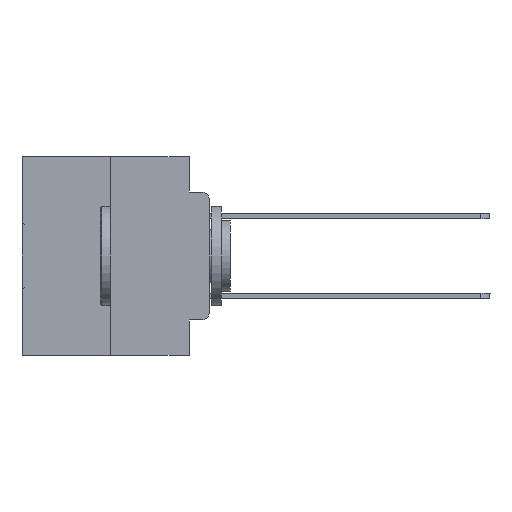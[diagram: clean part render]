
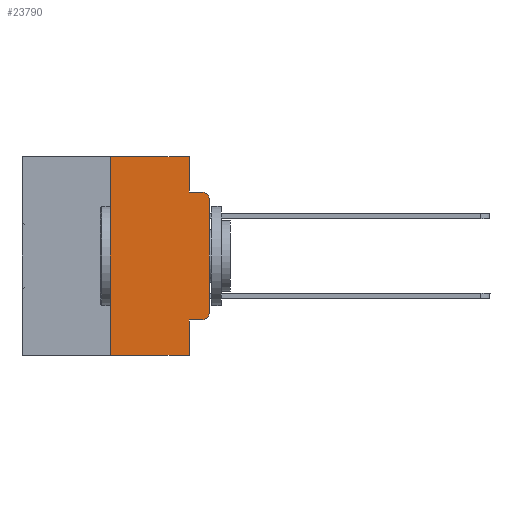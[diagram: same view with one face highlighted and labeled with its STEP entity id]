
A CAD part, left-side view. The second image highlights one B-rep face of the part: STEP entity #23790.
In plain terms, the highlighted planar face has unit normal (-1, 0, 0).
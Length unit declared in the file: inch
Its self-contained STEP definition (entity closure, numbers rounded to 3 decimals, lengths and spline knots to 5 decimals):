
#3 = VERTEX_POINT ( 'NONE', #14954 ) ;
#69 = ORIENTED_EDGE ( 'NONE', *, *, #8467, .T. ) ;
#255 = CARTESIAN_POINT ( 'NONE',  ( 0., 0.25, 0. ) ) ;
#316 = CARTESIAN_POINT ( 'NONE',  ( 0., 0.02, -0.3915 ) ) ;
#676 = EDGE_CURVE ( 'NONE', #5195, #7678, #20187, .T. ) ;
#709 = CARTESIAN_POINT ( 'NONE',  ( 0., 0.02, -0.0885 ) ) ;
#1615 = LINE ( 'NONE', #7010, #13814 ) ;
#2906 = VECTOR ( 'NONE', #10260, 39.37008 ) ;
#2927 = CARTESIAN_POINT ( 'NONE',  ( 0., 0.051, -0.4115 ) ) ;
#3789 = AXIS2_PLACEMENT_3D ( 'NONE', #316, #27270, #6475 ) ;
#3833 = DIRECTION ( 'NONE',  ( 1., 0., 0. ) ) ;
#3973 = EDGE_CURVE ( 'NONE', #9567, #18246, #27916, .T. ) ;
#4090 = EDGE_CURVE ( 'NONE', #33981, #18246, #19325, .T. ) ;
#4239 = EDGE_LOOP ( 'NONE', ( #30307, #14714, #23912, #22404, #26492, #5807, #30471, #18160, #69, #4255 ) ) ;
#4255 = ORIENTED_EDGE ( 'NONE', *, *, #676, .T. ) ;
#5195 = VERTEX_POINT ( 'NONE', #33158 ) ;
#5348 = LINE ( 'NONE', #20904, #2906 ) ;
#5396 = AXIS2_PLACEMENT_3D ( 'NONE', #18741, #26130, #15619 ) ;
#5807 = ORIENTED_EDGE ( 'NONE', *, *, #30444, .F. ) ;
#5916 = CARTESIAN_POINT ( 'NONE',  ( 0., 0.473, 0. ) ) ;
#6094 = DIRECTION ( 'NONE',  ( 0., 0., -1. ) ) ;
#6273 = EDGE_CURVE ( 'NONE', #7678, #33981, #1615, .T. ) ;
#6424 = CARTESIAN_POINT ( 'NONE',  ( 0., 0., -0.1085 ) ) ;
#6475 = DIRECTION ( 'NONE',  ( 0., 0., -1. ) ) ;
#7010 = CARTESIAN_POINT ( 'NONE',  ( 0., 0., 0. ) ) ;
#7244 = CARTESIAN_POINT ( 'NONE',  ( 0., 0.051, 0. ) ) ;
#7501 = LINE ( 'NONE', #28876, #15876 ) ;
#7605 = DIRECTION ( 'NONE',  ( 0., 0., 1. ) ) ;
#7678 = VERTEX_POINT ( 'NONE', #19292 ) ;
#8467 = EDGE_CURVE ( 'NONE', #31518, #5195, #26892, .T. ) ;
#8508 = CARTESIAN_POINT ( 'NONE',  ( 0., 0.051, -0.4115 ) ) ;
#9567 = VERTEX_POINT ( 'NONE', #23445 ) ;
#10260 = DIRECTION ( 'NONE',  ( 0., -1., 0. ) ) ;
#10972 = DIRECTION ( 'NONE',  ( 0., -1., 0. ) ) ;
#11409 = VECTOR ( 'NONE', #33988, 39.37008 ) ;
#11615 = VERTEX_POINT ( 'NONE', #28752 ) ;
#12507 = VECTOR ( 'NONE', #20404, 39.37008 ) ;
#12543 = CARTESIAN_POINT ( 'NONE',  ( 0., 0.051, 0. ) ) ;
#12655 = AXIS2_PLACEMENT_3D ( 'NONE', #5916, #3833, #6094 ) ;
#12841 = CARTESIAN_POINT ( 'NONE',  ( 0., 0.051, -0.5 ) ) ;
#13814 = VECTOR ( 'NONE', #17333, 39.37008 ) ;
#14016 = EDGE_CURVE ( 'NONE', #11615, #25646, #5348, .T. ) ;
#14714 = ORIENTED_EDGE ( 'NONE', *, *, #4090, .T. ) ;
#14954 = CARTESIAN_POINT ( 'NONE',  ( 0., 0.25, -0.5 ) ) ;
#15427 = VECTOR ( 'NONE', #20348, 39.37008 ) ;
#15507 = VECTOR ( 'NONE', #10972, 39.37008 ) ;
#15619 = DIRECTION ( 'NONE',  ( 0., 0., -1. ) ) ;
#15876 = VECTOR ( 'NONE', #29047, 39.37008 ) ;
#17333 = DIRECTION ( 'NONE',  ( 0., 0., 1. ) ) ;
#18160 = ORIENTED_EDGE ( 'NONE', *, *, #18769, .F. ) ;
#18246 = VERTEX_POINT ( 'NONE', #709 ) ;
#18741 = CARTESIAN_POINT ( 'NONE',  ( 0., 0.02, -0.1085 ) ) ;
#18769 = EDGE_CURVE ( 'NONE', #31518, #22701, #31112, .T. ) ;
#19173 = EDGE_CURVE ( 'NONE', #3, #22701, #33812, .T. ) ;
#19292 = CARTESIAN_POINT ( 'NONE',  ( 0., 0., -0.3915 ) ) ;
#19325 = CIRCLE ( 'NONE', #5396, 0.02 ) ;
#20187 = CIRCLE ( 'NONE', #3789, 0.02 ) ;
#20348 = DIRECTION ( 'NONE',  ( 0., -1., 0. ) ) ;
#20404 = DIRECTION ( 'NONE',  ( 0., 0., -1. ) ) ;
#20904 = CARTESIAN_POINT ( 'NONE',  ( 0., 0.473, 0. ) ) ;
#22404 = ORIENTED_EDGE ( 'NONE', *, *, #33691, .F. ) ;
#22701 = VERTEX_POINT ( 'NONE', #12841 ) ;
#22807 = CARTESIAN_POINT ( 'NONE',  ( 0., 0.051, -0.0885 ) ) ;
#23445 = CARTESIAN_POINT ( 'NONE',  ( 0., 0.051, -0.0885 ) ) ;
#23771 = FACE_OUTER_BOUND ( 'NONE', #4239, .T. ) ;
#23790 = ADVANCED_FACE ( 'NONE', ( #23771 ), #34468, .F. ) ;
#23912 = ORIENTED_EDGE ( 'NONE', *, *, #3973, .F. ) ;
#25646 = VERTEX_POINT ( 'NONE', #7244 ) ;
#26130 = DIRECTION ( 'NONE',  ( -1., 0., 0. ) ) ;
#26492 = ORIENTED_EDGE ( 'NONE', *, *, #14016, .F. ) ;
#26509 = LINE ( 'NONE', #255, #27479 ) ;
#26892 = LINE ( 'NONE', #2927, #15507 ) ;
#27270 = DIRECTION ( 'NONE',  ( -1., 0., 0. ) ) ;
#27479 = VECTOR ( 'NONE', #7605, 39.37008 ) ;
#27916 = LINE ( 'NONE', #22807, #15427 ) ;
#28744 = CARTESIAN_POINT ( 'NONE',  ( 0., 0.473, -0.5 ) ) ;
#28752 = CARTESIAN_POINT ( 'NONE',  ( 0., 0.25, 0. ) ) ;
#28876 = CARTESIAN_POINT ( 'NONE',  ( 0., 0.051, 0. ) ) ;
#29047 = DIRECTION ( 'NONE',  ( 0., 0., -1. ) ) ;
#30307 = ORIENTED_EDGE ( 'NONE', *, *, #6273, .T. ) ;
#30444 = EDGE_CURVE ( 'NONE', #3, #11615, #26509, .T. ) ;
#30471 = ORIENTED_EDGE ( 'NONE', *, *, #19173, .T. ) ;
#31112 = LINE ( 'NONE', #12543, #12507 ) ;
#31518 = VERTEX_POINT ( 'NONE', #8508 ) ;
#33158 = CARTESIAN_POINT ( 'NONE',  ( 0., 0.02, -0.4115 ) ) ;
#33691 = EDGE_CURVE ( 'NONE', #25646, #9567, #7501, .T. ) ;
#33812 = LINE ( 'NONE', #28744, #11409 ) ;
#33981 = VERTEX_POINT ( 'NONE', #6424 ) ;
#33988 = DIRECTION ( 'NONE',  ( 0., -1., 0. ) ) ;
#34468 = PLANE ( 'NONE',  #12655 ) ;
